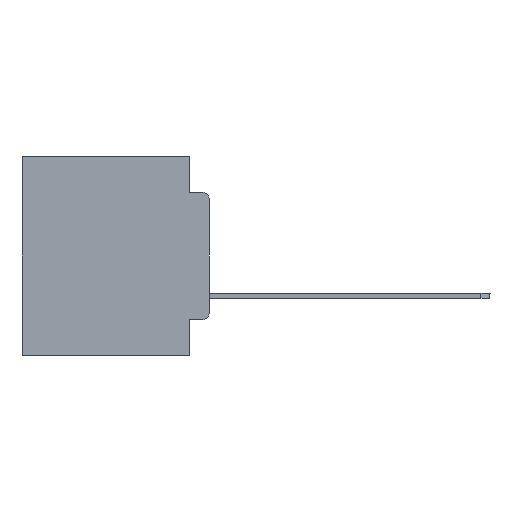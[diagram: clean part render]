
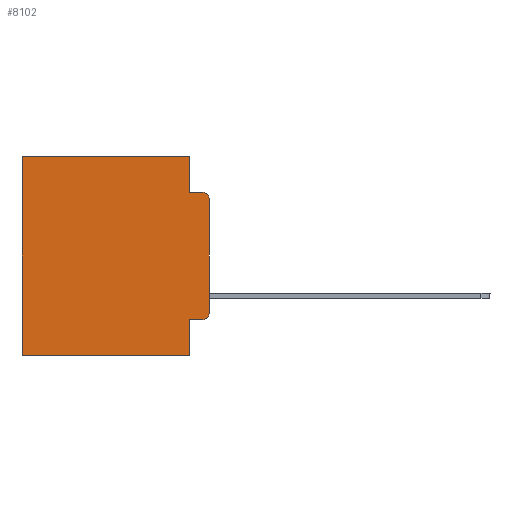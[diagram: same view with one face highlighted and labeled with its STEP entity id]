
A CAD part, left-side view. The second image highlights one B-rep face of the part: STEP entity #8102.
In plain terms, the highlighted planar face has unit normal (-1, 0, 0).
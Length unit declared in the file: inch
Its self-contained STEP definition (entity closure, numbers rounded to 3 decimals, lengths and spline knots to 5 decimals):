
#422 = DIRECTION ( 'NONE',  ( 0., -1., 0. ) ) ;
#529 = CARTESIAN_POINT ( 'NONE',  ( 0.298, 0., -0.5 ) ) ;
#896 = LINE ( 'NONE', #529, #26082 ) ;
#975 = DIRECTION ( 'NONE',  ( 0., 0., -1. ) ) ;
#1245 = DIRECTION ( 'NONE',  ( 0., 0., -1. ) ) ;
#1267 = EDGE_CURVE ( 'NONE', #22379, #5169, #26027, .T. ) ;
#1494 = AXIS2_PLACEMENT_3D ( 'NONE', #7971, #3224, #7762 ) ;
#1640 = VECTOR ( 'NONE', #422, 39.37008 ) ;
#1830 = CARTESIAN_POINT ( 'NONE',  ( 0.298, 0.051, -0.5 ) ) ;
#2105 = CARTESIAN_POINT ( 'NONE',  ( 0.298, 0.02, -0.4115 ) ) ;
#2217 = ORIENTED_EDGE ( 'NONE', *, *, #4020, .F. ) ;
#2398 = ORIENTED_EDGE ( 'NONE', *, *, #21690, .F. ) ;
#3224 = DIRECTION ( 'NONE',  ( 1., 0., 0. ) ) ;
#3359 = DIRECTION ( 'NONE',  ( -1., 0., 0. ) ) ;
#3920 = FACE_OUTER_BOUND ( 'NONE', #26476, .T. ) ;
#4020 = EDGE_CURVE ( 'NONE', #22845, #5169, #13587, .T. ) ;
#4168 = VERTEX_POINT ( 'NONE', #6301 ) ;
#4661 = ORIENTED_EDGE ( 'NONE', *, *, #1267, .T. ) ;
#4714 = DIRECTION ( 'NONE',  ( 0., 0., -1. ) ) ;
#5169 = VERTEX_POINT ( 'NONE', #27043 ) ;
#5446 = PLANE ( 'NONE',  #1494 ) ;
#5891 = CARTESIAN_POINT ( 'NONE',  ( 0.298, 0.051, -0.0885 ) ) ;
#6076 = DIRECTION ( 'NONE',  ( 0., 1., 0. ) ) ;
#6301 = CARTESIAN_POINT ( 'NONE',  ( 0.298, 0.051, 0. ) ) ;
#6351 = VECTOR ( 'NONE', #6076, 39.37008 ) ;
#6501 = CARTESIAN_POINT ( 'NONE',  ( 0.298, 0.02, -0.0885 ) ) ;
#6893 = VERTEX_POINT ( 'NONE', #28847 ) ;
#7158 = VECTOR ( 'NONE', #19799, 39.37008 ) ;
#7412 = ORIENTED_EDGE ( 'NONE', *, *, #27315, .F. ) ;
#7417 = VECTOR ( 'NONE', #4714, 39.37008 ) ;
#7485 = EDGE_CURVE ( 'NONE', #6893, #25703, #13560, .T. ) ;
#7762 = DIRECTION ( 'NONE',  ( 0., 0., -1. ) ) ;
#7971 = CARTESIAN_POINT ( 'NONE',  ( 0.298, 0., 0. ) ) ;
#8102 = ADVANCED_FACE ( 'NONE', ( #3920 ), #5446, .F. ) ;
#8380 = ORIENTED_EDGE ( 'NONE', *, *, #13862, .T. ) ;
#9205 = CARTESIAN_POINT ( 'NONE',  ( 0.298, 0., 0. ) ) ;
#9479 = DIRECTION ( 'NONE',  ( 0., 0., -1. ) ) ;
#10147 = ORIENTED_EDGE ( 'NONE', *, *, #27216, .T. ) ;
#10189 = LINE ( 'NONE', #12514, #20589 ) ;
#10316 = EDGE_CURVE ( 'NONE', #23825, #20383, #12126, .T. ) ;
#10486 = CARTESIAN_POINT ( 'NONE',  ( 0.298, 0.051, -0.0885 ) ) ;
#10640 = AXIS2_PLACEMENT_3D ( 'NONE', #17141, #3359, #24083 ) ;
#11208 = CARTESIAN_POINT ( 'NONE',  ( 0.298, 0.051, 0. ) ) ;
#12113 = EDGE_CURVE ( 'NONE', #22845, #20383, #26478, .T. ) ;
#12126 = LINE ( 'NONE', #10486, #7158 ) ;
#12395 = LINE ( 'NONE', #12943, #6351 ) ;
#12411 = DIRECTION ( 'NONE',  ( 0., 0., -1. ) ) ;
#12514 = CARTESIAN_POINT ( 'NONE',  ( 0.298, 0.473, 0. ) ) ;
#12943 = CARTESIAN_POINT ( 'NONE',  ( 0.298, 0., 0. ) ) ;
#13560 = LINE ( 'NONE', #19334, #26173 ) ;
#13587 = LINE ( 'NONE', #9205, #25133 ) ;
#13862 = EDGE_CURVE ( 'NONE', #16380, #18522, #10189, .T. ) ;
#16380 = VERTEX_POINT ( 'NONE', #19605 ) ;
#16484 = CARTESIAN_POINT ( 'NONE',  ( 0.298, 0.473, -0.5 ) ) ;
#17141 = CARTESIAN_POINT ( 'NONE',  ( 0.298, 0.02, -0.3915 ) ) ;
#18522 = VERTEX_POINT ( 'NONE', #16484 ) ;
#18754 = ORIENTED_EDGE ( 'NONE', *, *, #22178, .T. ) ;
#18889 = ORIENTED_EDGE ( 'NONE', *, *, #7485, .F. ) ;
#19334 = CARTESIAN_POINT ( 'NONE',  ( 0.298, 0.051, 0. ) ) ;
#19605 = CARTESIAN_POINT ( 'NONE',  ( 0.298, 0.473, 0. ) ) ;
#19799 = DIRECTION ( 'NONE',  ( 0., -1., 0. ) ) ;
#20383 = VERTEX_POINT ( 'NONE', #6501 ) ;
#20589 = VECTOR ( 'NONE', #12411, 39.37008 ) ;
#21690 = EDGE_CURVE ( 'NONE', #4168, #23825, #27237, .T. ) ;
#22178 = EDGE_CURVE ( 'NONE', #4168, #16380, #12395, .T. ) ;
#22379 = VERTEX_POINT ( 'NONE', #2105 ) ;
#22845 = VERTEX_POINT ( 'NONE', #27647 ) ;
#23825 = VERTEX_POINT ( 'NONE', #5891 ) ;
#24083 = DIRECTION ( 'NONE',  ( 0., 0., -1. ) ) ;
#24646 = LINE ( 'NONE', #27726, #1640 ) ;
#24915 = ORIENTED_EDGE ( 'NONE', *, *, #12113, .T. ) ;
#25133 = VECTOR ( 'NONE', #9479, 39.37008 ) ;
#25508 = AXIS2_PLACEMENT_3D ( 'NONE', #28358, #28559, #975 ) ;
#25703 = VERTEX_POINT ( 'NONE', #1830 ) ;
#25822 = ORIENTED_EDGE ( 'NONE', *, *, #10316, .F. ) ;
#26027 = CIRCLE ( 'NONE', #10640, 0.02 ) ;
#26082 = VECTOR ( 'NONE', #28219, 39.37008 ) ;
#26173 = VECTOR ( 'NONE', #1245, 39.37008 ) ;
#26476 = EDGE_LOOP ( 'NONE', ( #2217, #24915, #25822, #2398, #18754, #8380, #7412, #18889, #10147, #4661 ) ) ;
#26478 = CIRCLE ( 'NONE', #25508, 0.02 ) ;
#27043 = CARTESIAN_POINT ( 'NONE',  ( 0.298, 0., -0.3915 ) ) ;
#27216 = EDGE_CURVE ( 'NONE', #6893, #22379, #24646, .T. ) ;
#27237 = LINE ( 'NONE', #11208, #7417 ) ;
#27315 = EDGE_CURVE ( 'NONE', #25703, #18522, #896, .T. ) ;
#27647 = CARTESIAN_POINT ( 'NONE',  ( 0.298, 0., -0.1085 ) ) ;
#27726 = CARTESIAN_POINT ( 'NONE',  ( 0.298, 0.051, -0.4115 ) ) ;
#28219 = DIRECTION ( 'NONE',  ( 0., 1., 0. ) ) ;
#28358 = CARTESIAN_POINT ( 'NONE',  ( 0.298, 0.02, -0.1085 ) ) ;
#28559 = DIRECTION ( 'NONE',  ( -1., 0., 0. ) ) ;
#28847 = CARTESIAN_POINT ( 'NONE',  ( 0.298, 0.051, -0.4115 ) ) ;
